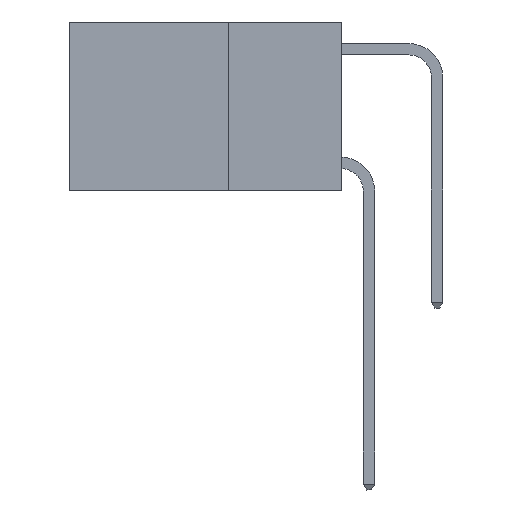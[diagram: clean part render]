
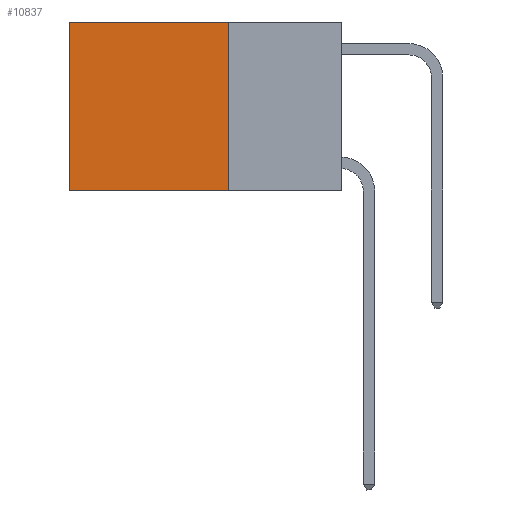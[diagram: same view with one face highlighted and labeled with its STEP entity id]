
A CAD part, left-side view. The second image highlights one B-rep face of the part: STEP entity #10837.
In plain terms, the highlighted planar face has unit normal (-1, 0, 0).
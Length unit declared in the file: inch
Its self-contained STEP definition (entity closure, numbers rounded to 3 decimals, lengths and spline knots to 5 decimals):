
#170 = DIRECTION ( 'NONE',  ( 0., 0., -1. ) ) ;
#713 = CARTESIAN_POINT ( 'NONE',  ( 0.2625, 0.25, 0. ) ) ;
#1102 = CARTESIAN_POINT ( 'NONE',  ( 0.2625, 0.6, -0.37 ) ) ;
#1108 = VERTEX_POINT ( 'NONE', #6599 ) ;
#1135 = AXIS2_PLACEMENT_3D ( 'NONE', #713, #4091, #10982 ) ;
#1248 = ORIENTED_EDGE ( 'NONE', *, *, #5482, .F. ) ;
#1492 = CARTESIAN_POINT ( 'NONE',  ( 0.2625, 0.6, 0. ) ) ;
#1498 = VERTEX_POINT ( 'NONE', #1102 ) ;
#1817 = VECTOR ( 'NONE', #170, 39.37008 ) ;
#2551 = VERTEX_POINT ( 'NONE', #8109 ) ;
#2675 = LINE ( 'NONE', #4502, #1817 ) ;
#2794 = ORIENTED_EDGE ( 'NONE', *, *, #10134, .T. ) ;
#2981 = EDGE_LOOP ( 'NONE', ( #2794, #1248, #5421, #9702 ) ) ;
#3713 = CARTESIAN_POINT ( 'NONE',  ( 0.2625, 0.25, -0.37 ) ) ;
#4091 = DIRECTION ( 'NONE',  ( 1., 0., 0. ) ) ;
#4455 = LINE ( 'NONE', #9396, #7215 ) ;
#4502 = CARTESIAN_POINT ( 'NONE',  ( 0.2625, 0.6, 0. ) ) ;
#4777 = LINE ( 'NONE', #8930, #7659 ) ;
#5101 = FACE_OUTER_BOUND ( 'NONE', #2981, .T. ) ;
#5421 = ORIENTED_EDGE ( 'NONE', *, *, #8670, .F. ) ;
#5482 = EDGE_CURVE ( 'NONE', #2551, #1498, #8680, .T. ) ;
#6599 = CARTESIAN_POINT ( 'NONE',  ( 0.2625, 0.25, 0. ) ) ;
#6641 = VERTEX_POINT ( 'NONE', #1492 ) ;
#7148 = EDGE_CURVE ( 'NONE', #1108, #6641, #4455, .T. ) ;
#7215 = VECTOR ( 'NONE', #7852, 39.37008 ) ;
#7239 = VECTOR ( 'NONE', #10590, 39.37008 ) ;
#7659 = VECTOR ( 'NONE', #8183, 39.37008 ) ;
#7852 = DIRECTION ( 'NONE',  ( 0., 1., 0. ) ) ;
#8109 = CARTESIAN_POINT ( 'NONE',  ( 0.2625, 0.25, -0.37 ) ) ;
#8183 = DIRECTION ( 'NONE',  ( 0., 0., -1. ) ) ;
#8446 = PLANE ( 'NONE',  #1135 ) ;
#8670 = EDGE_CURVE ( 'NONE', #1108, #2551, #4777, .T. ) ;
#8680 = LINE ( 'NONE', #3713, #7239 ) ;
#8930 = CARTESIAN_POINT ( 'NONE',  ( 0.2625, 0.25, 0. ) ) ;
#9396 = CARTESIAN_POINT ( 'NONE',  ( 0.2625, 0.25, 0. ) ) ;
#9702 = ORIENTED_EDGE ( 'NONE', *, *, #7148, .T. ) ;
#10134 = EDGE_CURVE ( 'NONE', #6641, #1498, #2675, .T. ) ;
#10590 = DIRECTION ( 'NONE',  ( 0., 1., 0. ) ) ;
#10837 = ADVANCED_FACE ( 'NONE', ( #5101 ), #8446, .F. ) ;
#10982 = DIRECTION ( 'NONE',  ( 0., 0., -1. ) ) ;
